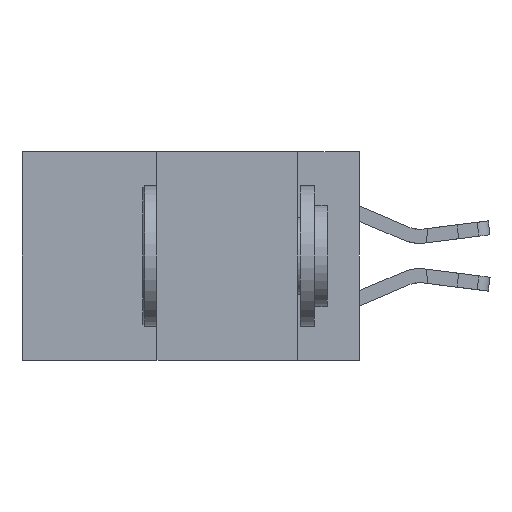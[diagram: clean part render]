
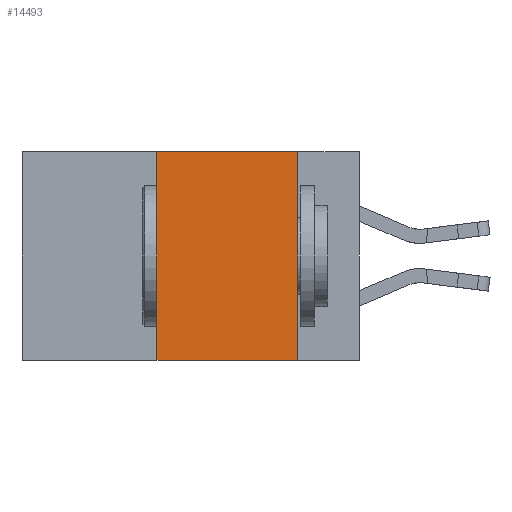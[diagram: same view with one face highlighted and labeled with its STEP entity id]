
A CAD part, left-side view. The second image highlights one B-rep face of the part: STEP entity #14493.
In plain terms, the highlighted planar face has unit normal (-1, 0, 0).
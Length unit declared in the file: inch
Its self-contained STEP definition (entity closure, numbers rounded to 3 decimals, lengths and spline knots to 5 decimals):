
#496 = LINE ( 'NONE', #548, #24234 ) ;
#542 = EDGE_CURVE ( 'NONE', #9015, #25272, #571, .T. ) ;
#548 = CARTESIAN_POINT ( 'NONE',  ( 0., 0.6, 0. ) ) ;
#571 = LINE ( 'NONE', #12310, #26472 ) ;
#814 = AXIS2_PLACEMENT_3D ( 'NONE', #9333, #25680, #21757 ) ;
#935 = EDGE_LOOP ( 'NONE', ( #5612, #22935, #21240, #27161 ) ) ;
#3921 = CARTESIAN_POINT ( 'NONE',  ( 0., 0.36, -0.37 ) ) ;
#4003 = EDGE_CURVE ( 'NONE', #25272, #11102, #496, .T. ) ;
#4103 = FACE_OUTER_BOUND ( 'NONE', #935, .T. ) ;
#4998 = CARTESIAN_POINT ( 'NONE',  ( 0., 0.11, 0. ) ) ;
#5612 = ORIENTED_EDGE ( 'NONE', *, *, #24132, .F. ) ;
#5829 = VECTOR ( 'NONE', #21284, 39.37008 ) ;
#6783 = EDGE_CURVE ( 'NONE', #9015, #17126, #28455, .T. ) ;
#6797 = CARTESIAN_POINT ( 'NONE',  ( 0., 0.6, -0.37 ) ) ;
#9015 = VERTEX_POINT ( 'NONE', #3921 ) ;
#9333 = CARTESIAN_POINT ( 'NONE',  ( 0., 0.6, 0. ) ) ;
#11102 = VERTEX_POINT ( 'NONE', #20595 ) ;
#12310 = CARTESIAN_POINT ( 'NONE',  ( 0., 0.36, 0. ) ) ;
#13127 = LINE ( 'NONE', #4998, #5829 ) ;
#13241 = PLANE ( 'NONE',  #814 ) ;
#14493 = ADVANCED_FACE ( 'NONE', ( #4103 ), #13241, .F. ) ;
#17126 = VERTEX_POINT ( 'NONE', #27313 ) ;
#18511 = DIRECTION ( 'NONE',  ( 0., -1., 0. ) ) ;
#18581 = CARTESIAN_POINT ( 'NONE',  ( 0., 0.36, 0. ) ) ;
#20595 = CARTESIAN_POINT ( 'NONE',  ( 0., 0.11, 0. ) ) ;
#21240 = ORIENTED_EDGE ( 'NONE', *, *, #542, .F. ) ;
#21284 = DIRECTION ( 'NONE',  ( 0., 0., -1. ) ) ;
#21706 = DIRECTION ( 'NONE',  ( 0., 0., 1. ) ) ;
#21757 = DIRECTION ( 'NONE',  ( 0., 0., -1. ) ) ;
#22935 = ORIENTED_EDGE ( 'NONE', *, *, #4003, .F. ) ;
#23585 = DIRECTION ( 'NONE',  ( 0., -1., 0. ) ) ;
#24132 = EDGE_CURVE ( 'NONE', #11102, #17126, #13127, .T. ) ;
#24234 = VECTOR ( 'NONE', #23585, 39.37008 ) ;
#25272 = VERTEX_POINT ( 'NONE', #18581 ) ;
#25680 = DIRECTION ( 'NONE',  ( 1., 0., 0. ) ) ;
#26472 = VECTOR ( 'NONE', #21706, 39.37008 ) ;
#27048 = VECTOR ( 'NONE', #18511, 39.37008 ) ;
#27161 = ORIENTED_EDGE ( 'NONE', *, *, #6783, .T. ) ;
#27313 = CARTESIAN_POINT ( 'NONE',  ( 0., 0.11, -0.37 ) ) ;
#28455 = LINE ( 'NONE', #6797, #27048 ) ;
